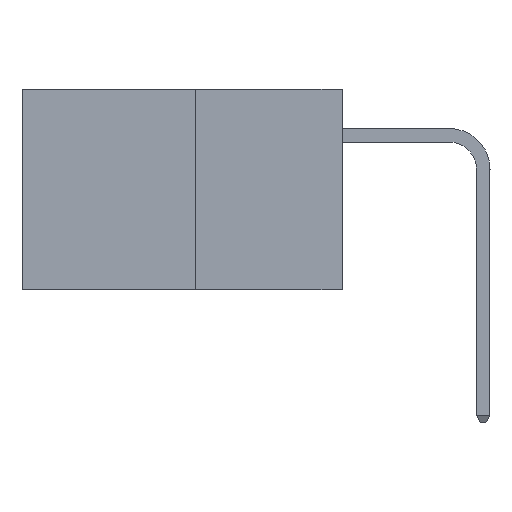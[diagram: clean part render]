
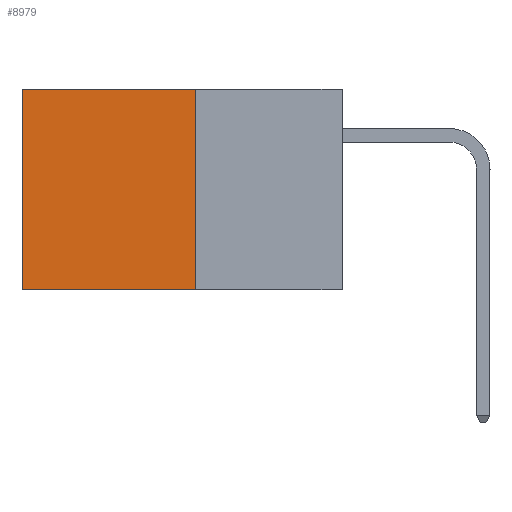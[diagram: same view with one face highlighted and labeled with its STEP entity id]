
A CAD part, left-side view. The second image highlights one B-rep face of the part: STEP entity #8979.
In plain terms, the highlighted planar face has unit normal (-1, 0, 0).
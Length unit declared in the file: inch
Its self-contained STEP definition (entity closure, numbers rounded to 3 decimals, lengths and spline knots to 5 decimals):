
#61 = CARTESIAN_POINT ( 'NONE',  ( 0.277, 0.59, -0.37 ) ) ;
#517 = LINE ( 'NONE', #12442, #9207 ) ;
#1674 = VECTOR ( 'NONE', #20182, 39.37008 ) ;
#1689 = DIRECTION ( 'NONE',  ( 0., 1., 0. ) ) ;
#2566 = CARTESIAN_POINT ( 'NONE',  ( 0.277, 0.27, -0.37 ) ) ;
#4401 = ORIENTED_EDGE ( 'NONE', *, *, #20778, .T. ) ;
#5159 = VERTEX_POINT ( 'NONE', #11427 ) ;
#5405 = VERTEX_POINT ( 'NONE', #8283 ) ;
#5941 = PLANE ( 'NONE',  #15520 ) ;
#6693 = EDGE_CURVE ( 'NONE', #5159, #10081, #11244, .T. ) ;
#6977 = CARTESIAN_POINT ( 'NONE',  ( 0.277, 0.27, -0.37 ) ) ;
#7583 = ORIENTED_EDGE ( 'NONE', *, *, #6693, .F. ) ;
#7643 = DIRECTION ( 'NONE',  ( 1., 0., 0. ) ) ;
#8283 = CARTESIAN_POINT ( 'NONE',  ( 0.277, 0.59, 0. ) ) ;
#8979 = ADVANCED_FACE ( 'NONE', ( #12475 ), #5941, .F. ) ;
#9186 = LINE ( 'NONE', #20019, #17484 ) ;
#9207 = VECTOR ( 'NONE', #10711, 39.37008 ) ;
#10081 = VERTEX_POINT ( 'NONE', #61 ) ;
#10190 = VECTOR ( 'NONE', #12606, 39.37008 ) ;
#10711 = DIRECTION ( 'NONE',  ( 0., 0., -1. ) ) ;
#11244 = LINE ( 'NONE', #6977, #1674 ) ;
#11427 = CARTESIAN_POINT ( 'NONE',  ( 0.277, 0.27, -0.37 ) ) ;
#12442 = CARTESIAN_POINT ( 'NONE',  ( 0.277, 0.59, -0.37 ) ) ;
#12475 = FACE_OUTER_BOUND ( 'NONE', #18639, .T. ) ;
#12606 = DIRECTION ( 'NONE',  ( 0., 0., -1. ) ) ;
#14559 = VERTEX_POINT ( 'NONE', #18580 ) ;
#15520 = AXIS2_PLACEMENT_3D ( 'NONE', #20734, #7643, #19182 ) ;
#15994 = ORIENTED_EDGE ( 'NONE', *, *, #20321, .T. ) ;
#16164 = ORIENTED_EDGE ( 'NONE', *, *, #21675, .F. ) ;
#17484 = VECTOR ( 'NONE', #1689, 39.37008 ) ;
#18580 = CARTESIAN_POINT ( 'NONE',  ( 0.277, 0.27, 0. ) ) ;
#18639 = EDGE_LOOP ( 'NONE', ( #15994, #7583, #16164, #4401 ) ) ;
#18951 = LINE ( 'NONE', #2566, #10190 ) ;
#19182 = DIRECTION ( 'NONE',  ( 0., 0., -1. ) ) ;
#20019 = CARTESIAN_POINT ( 'NONE',  ( 0.277, 0.27, 0. ) ) ;
#20182 = DIRECTION ( 'NONE',  ( 0., 1., 0. ) ) ;
#20321 = EDGE_CURVE ( 'NONE', #5405, #10081, #517, .T. ) ;
#20734 = CARTESIAN_POINT ( 'NONE',  ( 0.277, 0.27, -0.37 ) ) ;
#20778 = EDGE_CURVE ( 'NONE', #14559, #5405, #9186, .T. ) ;
#21675 = EDGE_CURVE ( 'NONE', #14559, #5159, #18951, .T. ) ;
